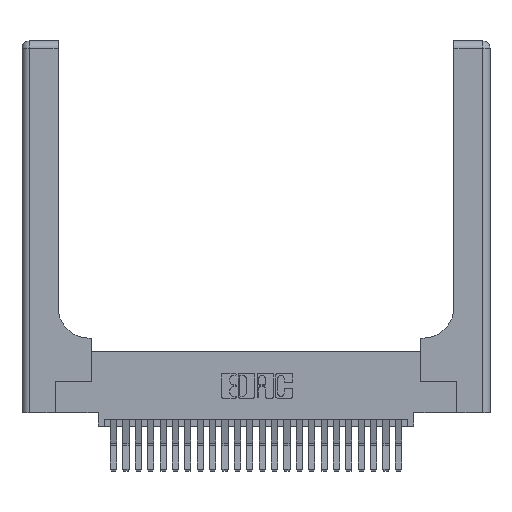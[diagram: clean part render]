
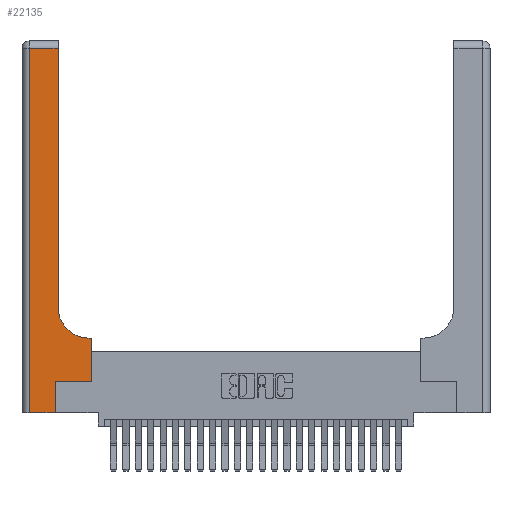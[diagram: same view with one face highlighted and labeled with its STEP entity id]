
A CAD part, top view. The second image highlights one B-rep face of the part: STEP entity #22135.
In plain terms, the highlighted planar face has unit normal (0, 0, 1).
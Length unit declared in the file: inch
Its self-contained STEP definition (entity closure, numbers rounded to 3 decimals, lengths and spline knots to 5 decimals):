
#250 = VERTEX_POINT ( 'NONE', #4092 ) ;
#619 = VECTOR ( 'NONE', #13869, 39.37008 ) ;
#999 = CARTESIAN_POINT ( 'NONE',  ( 0.2915, 0.85, 0.37 ) ) ;
#1258 = ORIENTED_EDGE ( 'NONE', *, *, #22886, .T. ) ;
#1575 = CARTESIAN_POINT ( 'NONE',  ( 0.269, 0., 0.37 ) ) ;
#1658 = VERTEX_POINT ( 'NONE', #2653 ) ;
#1955 = VECTOR ( 'NONE', #13853, 39.37008 ) ;
#2493 = VERTEX_POINT ( 'NONE', #999 ) ;
#2653 = CARTESIAN_POINT ( 'NONE',  ( 0.06, 2.94, 0.37 ) ) ;
#2904 = CARTESIAN_POINT ( 'NONE',  ( 0., 0., 0.37 ) ) ;
#3156 = EDGE_CURVE ( 'NONE', #2493, #9128, #19614, .T. ) ;
#3195 = EDGE_CURVE ( 'NONE', #7397, #21590, #24792, .T. ) ;
#3280 = EDGE_CURVE ( 'NONE', #16395, #250, #8658, .T. ) ;
#3597 = LINE ( 'NONE', #6703, #24212 ) ;
#3793 = CIRCLE ( 'NONE', #16059, 0.25 ) ;
#4073 = EDGE_CURVE ( 'NONE', #4506, #16395, #21536, .T. ) ;
#4092 = CARTESIAN_POINT ( 'NONE',  ( 0.5415, 0.6, 0.37 ) ) ;
#4132 = DIRECTION ( 'NONE',  ( -1., 0., 0. ) ) ;
#4178 = DIRECTION ( 'NONE',  ( 0., -1., 0. ) ) ;
#4194 = VECTOR ( 'NONE', #9791, 39.37008 ) ;
#4390 = ORIENTED_EDGE ( 'NONE', *, *, #19336, .T. ) ;
#4393 = EDGE_CURVE ( 'NONE', #21590, #4506, #16990, .T. ) ;
#4506 = VERTEX_POINT ( 'NONE', #10262 ) ;
#5583 = ORIENTED_EDGE ( 'NONE', *, *, #8021, .T. ) ;
#5794 = CARTESIAN_POINT ( 'NONE',  ( 0.2915, 3., 0.37 ) ) ;
#6015 = PLANE ( 'NONE',  #14203 ) ;
#6703 = CARTESIAN_POINT ( 'NONE',  ( 0., 2.94, 0.37 ) ) ;
#7121 = ORIENTED_EDGE ( 'NONE', *, *, #3195, .T. ) ;
#7397 = VERTEX_POINT ( 'NONE', #24979 ) ;
#7870 = ORIENTED_EDGE ( 'NONE', *, *, #3156, .T. ) ;
#8021 = EDGE_CURVE ( 'NONE', #250, #2493, #3793, .T. ) ;
#8252 = DIRECTION ( 'NONE',  ( 0., 1., 0. ) ) ;
#8658 = LINE ( 'NONE', #22256, #1955 ) ;
#9128 = VERTEX_POINT ( 'NONE', #13472 ) ;
#9215 = DIRECTION ( 'NONE',  ( 0., 0., -1. ) ) ;
#9791 = DIRECTION ( 'NONE',  ( 0., 1., 0. ) ) ;
#10079 = DIRECTION ( 'NONE',  ( 1., 0., 0. ) ) ;
#10262 = CARTESIAN_POINT ( 'NONE',  ( 0.5585, 0.25, 0.37 ) ) ;
#11151 = VERTEX_POINT ( 'NONE', #12822 ) ;
#11962 = ORIENTED_EDGE ( 'NONE', *, *, #4393, .T. ) ;
#12822 = CARTESIAN_POINT ( 'NONE',  ( 0.06, 0., 0.37 ) ) ;
#13472 = CARTESIAN_POINT ( 'NONE',  ( 0.2915, 2.94, 0.37 ) ) ;
#13853 = DIRECTION ( 'NONE',  ( -1., 0., 0. ) ) ;
#13869 = DIRECTION ( 'NONE',  ( 1., 0., 0. ) ) ;
#14203 = AXIS2_PLACEMENT_3D ( 'NONE', #16331, #26570, #4132 ) ;
#14420 = VECTOR ( 'NONE', #8252, 39.37008 ) ;
#16059 = AXIS2_PLACEMENT_3D ( 'NONE', #17442, #9215, #17606 ) ;
#16216 = CARTESIAN_POINT ( 'NONE',  ( 0.269, 0.25, 0.37 ) ) ;
#16223 = ORIENTED_EDGE ( 'NONE', *, *, #3280, .T. ) ;
#16331 = CARTESIAN_POINT ( 'NONE',  ( 0., 3., 0.37 ) ) ;
#16395 = VERTEX_POINT ( 'NONE', #17263 ) ;
#16628 = LINE ( 'NONE', #2904, #21478 ) ;
#16888 = EDGE_LOOP ( 'NONE', ( #7870, #1258, #4390, #17631, #7121, #11962, #22479, #16223, #5583 ) ) ;
#16990 = LINE ( 'NONE', #16216, #619 ) ;
#17263 = CARTESIAN_POINT ( 'NONE',  ( 0.5585, 0.6, 0.37 ) ) ;
#17442 = CARTESIAN_POINT ( 'NONE',  ( 0.5415, 0.85, 0.37 ) ) ;
#17606 = DIRECTION ( 'NONE',  ( 1., 0., 0. ) ) ;
#17631 = ORIENTED_EDGE ( 'NONE', *, *, #21641, .T. ) ;
#18490 = CARTESIAN_POINT ( 'NONE',  ( 0.269, 0.25, 0.37 ) ) ;
#18746 = DIRECTION ( 'NONE',  ( -1., 0., 0. ) ) ;
#19336 = EDGE_CURVE ( 'NONE', #1658, #11151, #26627, .T. ) ;
#19614 = LINE ( 'NONE', #5794, #4194 ) ;
#20040 = FACE_OUTER_BOUND ( 'NONE', #16888, .T. ) ;
#20619 = CARTESIAN_POINT ( 'NONE',  ( 0.5585, 0.25, 0.37 ) ) ;
#20641 = CARTESIAN_POINT ( 'NONE',  ( 0.06, 3., 0.37 ) ) ;
#21434 = VECTOR ( 'NONE', #4178, 39.37008 ) ;
#21478 = VECTOR ( 'NONE', #10079, 39.37008 ) ;
#21536 = LINE ( 'NONE', #20619, #14420 ) ;
#21590 = VERTEX_POINT ( 'NONE', #18490 ) ;
#21641 = EDGE_CURVE ( 'NONE', #11151, #7397, #16628, .T. ) ;
#22135 = ADVANCED_FACE ( 'NONE', ( #20040 ), #6015, .F. ) ;
#22256 = CARTESIAN_POINT ( 'NONE',  ( 0.2915, 0.6, 0.37 ) ) ;
#22479 = ORIENTED_EDGE ( 'NONE', *, *, #4073, .T. ) ;
#22886 = EDGE_CURVE ( 'NONE', #9128, #1658, #3597, .T. ) ;
#23198 = VECTOR ( 'NONE', #26075, 39.37008 ) ;
#24212 = VECTOR ( 'NONE', #18746, 39.37008 ) ;
#24792 = LINE ( 'NONE', #1575, #23198 ) ;
#24979 = CARTESIAN_POINT ( 'NONE',  ( 0.269, 0., 0.37 ) ) ;
#26075 = DIRECTION ( 'NONE',  ( 0., 1., 0. ) ) ;
#26570 = DIRECTION ( 'NONE',  ( 0., 0., -1. ) ) ;
#26627 = LINE ( 'NONE', #20641, #21434 ) ;
